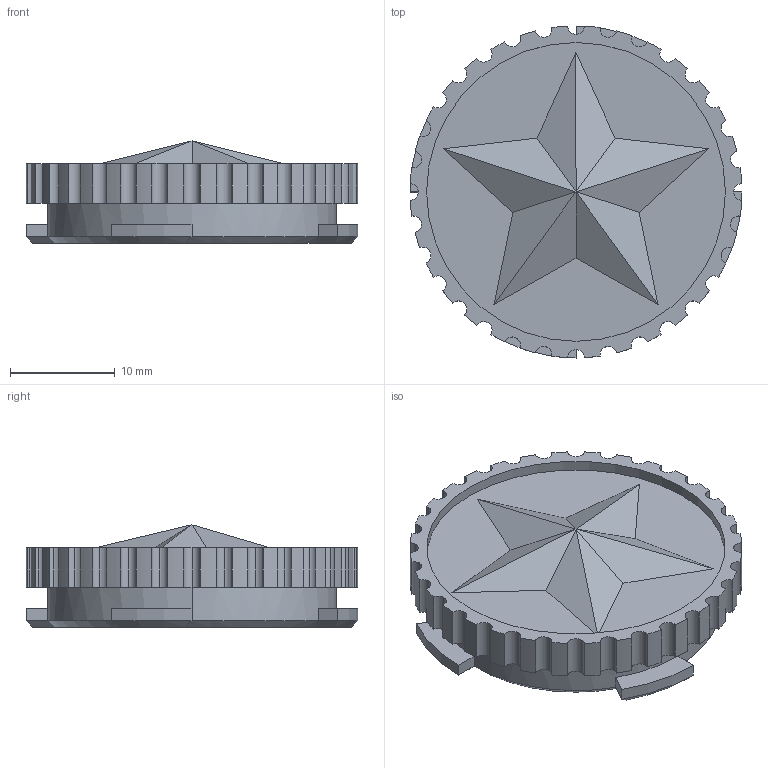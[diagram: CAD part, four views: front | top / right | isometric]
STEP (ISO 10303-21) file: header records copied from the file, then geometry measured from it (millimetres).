
FILE_DESCRIPTION (( 'STEP AP203' ), '1' );
FILE_NAME ('AF-HF-TK-PRT-001-STEP.STEP', '2020-12-04T13:11:36', ( '' ), ( '' ), 'SwSTEP 2.0', 'SolidWorks 2018', '' );
FILE_SCHEMA (( 'CONFIG_CONTROL_DESIGN' ));
Length unit declared in the file: inch
Products named in the file (1): AF-HF-TK-PRT-001-STEP
Bounding box: 31.75 x 31.75 x 9.79 mm (x, y, z)
Volume: 3924.1 mm3; surface area: 2674.6 mm2
Topology: 1 solids, 1 shells, 138 faces, 365 edges, 233 vertices
Faces by surface type: cylinder 89, plane 34, cone 13, sphere 2
Entity records: 4435 total; most frequent: DIRECTION 826, CARTESIAN_POINT 785, ORIENTED_EDGE 730, EDGE_CURVE 365, AXIS2_PLACEMENT_3D 338, VERTEX_POINT 233, CIRCLE 199, LINE 150
